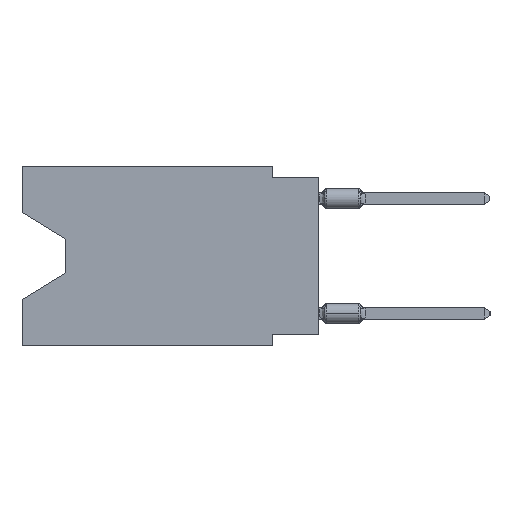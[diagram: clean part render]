
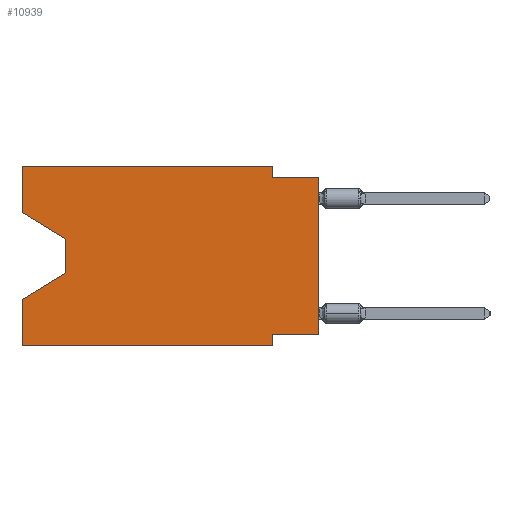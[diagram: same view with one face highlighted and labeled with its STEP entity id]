
A CAD part, left-side view. The second image highlights one B-rep face of the part: STEP entity #10939.
In plain terms, the highlighted planar face has unit normal (-1, 0, 0).
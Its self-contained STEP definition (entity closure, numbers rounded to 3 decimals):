
#472 = DIRECTION ( 'NONE',  ( 0., -0.855, -0.519 ) ) ;
#1551 = CARTESIAN_POINT ( 'NONE',  ( 0., 16.383, 0. ) ) ;
#1641 = VECTOR ( 'NONE', #28400, 1000. ) ;
#1933 = CARTESIAN_POINT ( 'NONE',  ( 0., 13.97, -5.893 ) ) ;
#2433 = DIRECTION ( 'NONE',  ( 0., 0., -1. ) ) ;
#2626 = CARTESIAN_POINT ( 'NONE',  ( 0., 2.54, -9.271 ) ) ;
#3155 = VECTOR ( 'NONE', #2433, 1000. ) ;
#3249 = VERTEX_POINT ( 'NONE', #30087 ) ;
#4087 = CARTESIAN_POINT ( 'NONE',  ( 0., 0., -9.271 ) ) ;
#4168 = CARTESIAN_POINT ( 'NONE',  ( 0., 16.383, 0. ) ) ;
#4224 = FACE_OUTER_BOUND ( 'NONE', #32558, .T. ) ;
#4484 = EDGE_CURVE ( 'NONE', #17251, #35358, #12603, .T. ) ;
#4609 = DIRECTION ( 'NONE',  ( 0., 0.855, -0.519 ) ) ;
#4753 = DIRECTION ( 'NONE',  ( 1., 0., 0. ) ) ;
#4785 = DIRECTION ( 'NONE',  ( 0., 0., -1. ) ) ;
#5151 = VERTEX_POINT ( 'NONE', #23152 ) ;
#5799 = ORIENTED_EDGE ( 'NONE', *, *, #17899, .F. ) ;
#5878 = EDGE_CURVE ( 'NONE', #22073, #9257, #16112, .T. ) ;
#7006 = VECTOR ( 'NONE', #23949, 1000. ) ;
#7547 = ORIENTED_EDGE ( 'NONE', *, *, #24251, .F. ) ;
#7698 = VECTOR ( 'NONE', #13622, 1000. ) ;
#7753 = LINE ( 'NONE', #32109, #13831 ) ;
#8099 = VERTEX_POINT ( 'NONE', #21618 ) ;
#8126 = EDGE_CURVE ( 'NONE', #8896, #3249, #8882, .T. ) ;
#8882 = LINE ( 'NONE', #25353, #29943 ) ;
#8896 = VERTEX_POINT ( 'NONE', #27396 ) ;
#9257 = VERTEX_POINT ( 'NONE', #2626 ) ;
#10312 = CARTESIAN_POINT ( 'NONE',  ( 0., 13.97, -4.013 ) ) ;
#10359 = LINE ( 'NONE', #10541, #34046 ) ;
#10541 = CARTESIAN_POINT ( 'NONE',  ( 0., 16.383, -9.906 ) ) ;
#10623 = DIRECTION ( 'NONE',  ( 0., 0., 1. ) ) ;
#10698 = LINE ( 'NONE', #21630, #7006 ) ;
#10939 = ADVANCED_FACE ( 'NONE', ( #4224 ), #15166, .F. ) ;
#11031 = EDGE_CURVE ( 'NONE', #3249, #28286, #35022, .T. ) ;
#12221 = VECTOR ( 'NONE', #4785, 1000. ) ;
#12603 = LINE ( 'NONE', #24049, #28760 ) ;
#12894 = ORIENTED_EDGE ( 'NONE', *, *, #11031, .T. ) ;
#12956 = VERTEX_POINT ( 'NONE', #17069 ) ;
#13059 = VECTOR ( 'NONE', #34128, 1000. ) ;
#13342 = ORIENTED_EDGE ( 'NONE', *, *, #28895, .F. ) ;
#13622 = DIRECTION ( 'NONE',  ( 0., 1., 0. ) ) ;
#13788 = DIRECTION ( 'NONE',  ( 0., -1., 0. ) ) ;
#13831 = VECTOR ( 'NONE', #10623, 1000. ) ;
#14166 = ORIENTED_EDGE ( 'NONE', *, *, #32601, .T. ) ;
#15166 = PLANE ( 'NONE',  #27839 ) ;
#15875 = VERTEX_POINT ( 'NONE', #19282 ) ;
#16112 = LINE ( 'NONE', #24883, #7698 ) ;
#16139 = ORIENTED_EDGE ( 'NONE', *, *, #8126, .T. ) ;
#16151 = EDGE_CURVE ( 'NONE', #22073, #8099, #7753, .T. ) ;
#17069 = CARTESIAN_POINT ( 'NONE',  ( 0., 2.54, -0.635 ) ) ;
#17251 = VERTEX_POINT ( 'NONE', #4168 ) ;
#17593 = ORIENTED_EDGE ( 'NONE', *, *, #27719, .F. ) ;
#17899 = EDGE_CURVE ( 'NONE', #8896, #17251, #18411, .T. ) ;
#18411 = LINE ( 'NONE', #27010, #19363 ) ;
#18766 = LINE ( 'NONE', #1933, #24177 ) ;
#19282 = CARTESIAN_POINT ( 'NONE',  ( 0., 2.54, -9.906 ) ) ;
#19363 = VECTOR ( 'NONE', #34886, 1000. ) ;
#19522 = CARTESIAN_POINT ( 'NONE',  ( 0., 2.54, -9.906 ) ) ;
#20178 = CARTESIAN_POINT ( 'NONE',  ( 0., 2.54, 0. ) ) ;
#20909 = ORIENTED_EDGE ( 'NONE', *, *, #4484, .F. ) ;
#21423 = DIRECTION ( 'NONE',  ( 0., 0., -1. ) ) ;
#21618 = CARTESIAN_POINT ( 'NONE',  ( 0., 0., -0.635 ) ) ;
#21630 = CARTESIAN_POINT ( 'NONE',  ( 0., 0., -0.635 ) ) ;
#22073 = VERTEX_POINT ( 'NONE', #4087 ) ;
#22274 = EDGE_CURVE ( 'NONE', #28286, #24359, #18766, .T. ) ;
#22860 = CARTESIAN_POINT ( 'NONE',  ( 0., 16.383, 0. ) ) ;
#23101 = ORIENTED_EDGE ( 'NONE', *, *, #22274, .T. ) ;
#23152 = CARTESIAN_POINT ( 'NONE',  ( 0., 16.383, -9.906 ) ) ;
#23205 = CARTESIAN_POINT ( 'NONE',  ( 0., 16.383, -7.36 ) ) ;
#23545 = LINE ( 'NONE', #22860, #1641 ) ;
#23949 = DIRECTION ( 'NONE',  ( 0., -1., 0. ) ) ;
#24049 = CARTESIAN_POINT ( 'NONE',  ( 0., 16.383, 0. ) ) ;
#24177 = VECTOR ( 'NONE', #4609, 1000. ) ;
#24251 = EDGE_CURVE ( 'NONE', #9257, #15875, #27576, .T. ) ;
#24359 = VERTEX_POINT ( 'NONE', #23205 ) ;
#24366 = ORIENTED_EDGE ( 'NONE', *, *, #5878, .F. ) ;
#24649 = EDGE_CURVE ( 'NONE', #5151, #24359, #23545, .T. ) ;
#24883 = CARTESIAN_POINT ( 'NONE',  ( 0., 0., -9.271 ) ) ;
#25353 = CARTESIAN_POINT ( 'NONE',  ( 0., 16.383, -2.546 ) ) ;
#26563 = DIRECTION ( 'NONE',  ( 0., -1., 0. ) ) ;
#27010 = CARTESIAN_POINT ( 'NONE',  ( 0., 16.383, 0. ) ) ;
#27396 = CARTESIAN_POINT ( 'NONE',  ( 0., 16.383, -2.546 ) ) ;
#27576 = LINE ( 'NONE', #19522, #13059 ) ;
#27719 = EDGE_CURVE ( 'NONE', #12956, #8099, #10698, .T. ) ;
#27839 = AXIS2_PLACEMENT_3D ( 'NONE', #1551, #4753, #21423 ) ;
#28286 = VERTEX_POINT ( 'NONE', #29986 ) ;
#28400 = DIRECTION ( 'NONE',  ( 0., 0., 1. ) ) ;
#28760 = VECTOR ( 'NONE', #26563, 1000. ) ;
#28895 = EDGE_CURVE ( 'NONE', #35358, #12956, #32375, .T. ) ;
#29675 = CARTESIAN_POINT ( 'NONE',  ( 0., 2.54, 0. ) ) ;
#29943 = VECTOR ( 'NONE', #472, 1000. ) ;
#29986 = CARTESIAN_POINT ( 'NONE',  ( 0., 13.97, -5.893 ) ) ;
#30087 = CARTESIAN_POINT ( 'NONE',  ( 0., 13.97, -4.013 ) ) ;
#30308 = ORIENTED_EDGE ( 'NONE', *, *, #16151, .T. ) ;
#32109 = CARTESIAN_POINT ( 'NONE',  ( 0., 0., 0. ) ) ;
#32375 = LINE ( 'NONE', #29675, #12221 ) ;
#32558 = EDGE_LOOP ( 'NONE', ( #16139, #12894, #23101, #33138, #14166, #7547, #24366, #30308, #17593, #13342, #20909, #5799 ) ) ;
#32601 = EDGE_CURVE ( 'NONE', #5151, #15875, #10359, .T. ) ;
#33138 = ORIENTED_EDGE ( 'NONE', *, *, #24649, .F. ) ;
#34046 = VECTOR ( 'NONE', #13788, 1000. ) ;
#34128 = DIRECTION ( 'NONE',  ( 0., 0., -1. ) ) ;
#34886 = DIRECTION ( 'NONE',  ( 0., 0., 1. ) ) ;
#35022 = LINE ( 'NONE', #10312, #3155 ) ;
#35358 = VERTEX_POINT ( 'NONE', #20178 ) ;
